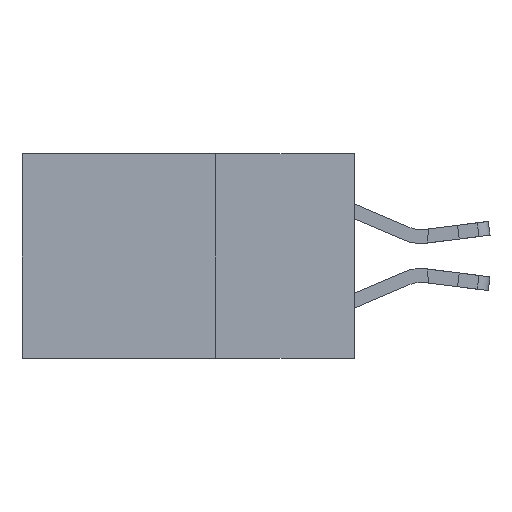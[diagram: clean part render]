
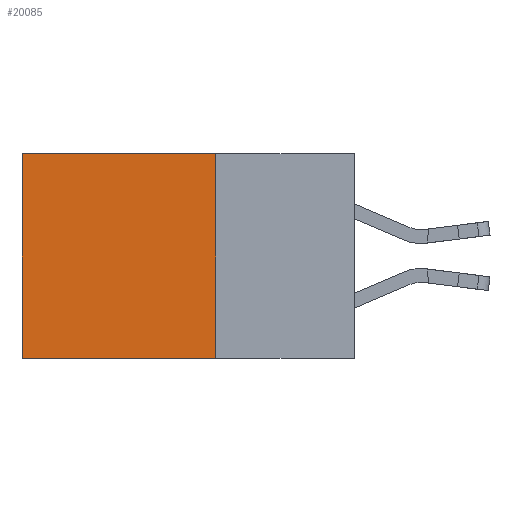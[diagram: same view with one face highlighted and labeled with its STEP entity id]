
A CAD part, left-side view. The second image highlights one B-rep face of the part: STEP entity #20085.
In plain terms, the highlighted planar face has unit normal (-1, 0, 0).
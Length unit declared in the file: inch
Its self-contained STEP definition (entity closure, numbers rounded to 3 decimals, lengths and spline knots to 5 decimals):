
#345 = EDGE_CURVE ( 'NONE', #1390, #21970, #389, .T. ) ;
#389 = LINE ( 'NONE', #4639, #998 ) ;
#998 = VECTOR ( 'NONE', #8183, 39.37008 ) ;
#1217 = LINE ( 'NONE', #1792, #10153 ) ;
#1309 = DIRECTION ( 'NONE',  ( 0., 1., 0. ) ) ;
#1390 = VERTEX_POINT ( 'NONE', #10985 ) ;
#1792 = CARTESIAN_POINT ( 'NONE',  ( 0.2615, 0.25, 0. ) ) ;
#2269 = CARTESIAN_POINT ( 'NONE',  ( 0.2615, 0.25, -0.37 ) ) ;
#2336 = VERTEX_POINT ( 'NONE', #6367 ) ;
#3731 = EDGE_LOOP ( 'NONE', ( #3759, #7042, #11675, #13040 ) ) ;
#3759 = ORIENTED_EDGE ( 'NONE', *, *, #7126, .T. ) ;
#4639 = CARTESIAN_POINT ( 'NONE',  ( 0.2615, 0.25, -0.37 ) ) ;
#4835 = DIRECTION ( 'NONE',  ( 1., 0., 0. ) ) ;
#6000 = VECTOR ( 'NONE', #16807, 39.37008 ) ;
#6367 = CARTESIAN_POINT ( 'NONE',  ( 0.2615, 0.6, 0. ) ) ;
#6889 = EDGE_CURVE ( 'NONE', #17699, #2336, #1217, .T. ) ;
#7042 = ORIENTED_EDGE ( 'NONE', *, *, #345, .F. ) ;
#7126 = EDGE_CURVE ( 'NONE', #2336, #21970, #18051, .T. ) ;
#8036 = FACE_OUTER_BOUND ( 'NONE', #3731, .T. ) ;
#8183 = DIRECTION ( 'NONE',  ( 0., 1., 0. ) ) ;
#9307 = VECTOR ( 'NONE', #11640, 39.37008 ) ;
#10002 = CARTESIAN_POINT ( 'NONE',  ( 0.2615, 0.6, -0.37 ) ) ;
#10153 = VECTOR ( 'NONE', #1309, 39.37008 ) ;
#10985 = CARTESIAN_POINT ( 'NONE',  ( 0.2615, 0.25, -0.37 ) ) ;
#11640 = DIRECTION ( 'NONE',  ( 0., 0., -1. ) ) ;
#11675 = ORIENTED_EDGE ( 'NONE', *, *, #22409, .F. ) ;
#11926 = CARTESIAN_POINT ( 'NONE',  ( 0.2615, 0.6, -0.37 ) ) ;
#13040 = ORIENTED_EDGE ( 'NONE', *, *, #6889, .T. ) ;
#15052 = AXIS2_PLACEMENT_3D ( 'NONE', #18742, #4835, #17091 ) ;
#16807 = DIRECTION ( 'NONE',  ( 0., 0., -1. ) ) ;
#17091 = DIRECTION ( 'NONE',  ( 0., 0., -1. ) ) ;
#17699 = VERTEX_POINT ( 'NONE', #21263 ) ;
#18051 = LINE ( 'NONE', #11926, #9307 ) ;
#18742 = CARTESIAN_POINT ( 'NONE',  ( 0.2615, 0.25, -0.37 ) ) ;
#19899 = LINE ( 'NONE', #2269, #6000 ) ;
#20085 = ADVANCED_FACE ( 'NONE', ( #8036 ), #22136, .F. ) ;
#21263 = CARTESIAN_POINT ( 'NONE',  ( 0.2615, 0.25, 0. ) ) ;
#21970 = VERTEX_POINT ( 'NONE', #10002 ) ;
#22136 = PLANE ( 'NONE',  #15052 ) ;
#22409 = EDGE_CURVE ( 'NONE', #17699, #1390, #19899, .T. ) ;
